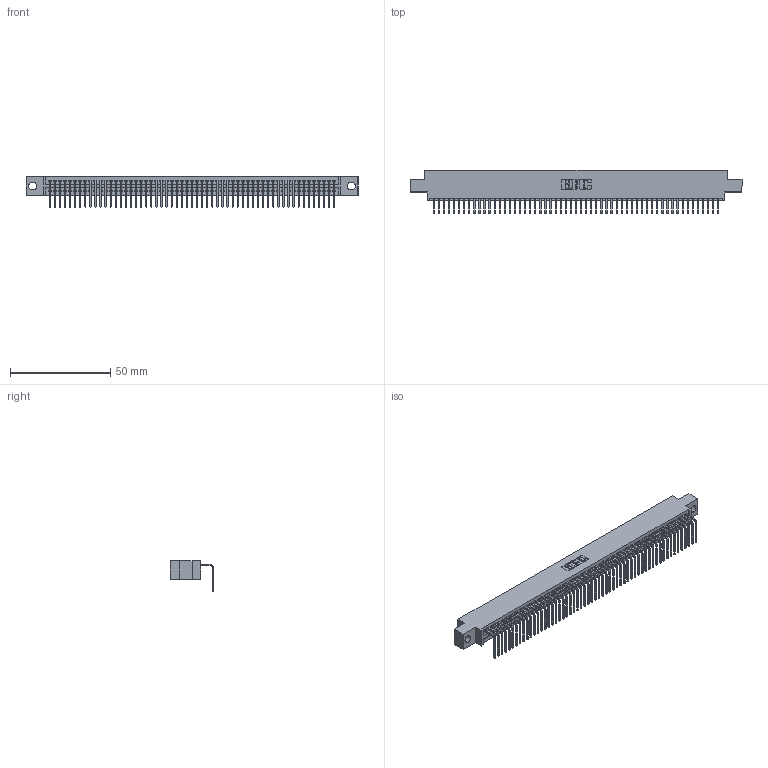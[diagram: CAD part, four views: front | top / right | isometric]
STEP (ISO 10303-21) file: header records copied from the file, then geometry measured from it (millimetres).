
FILE_DESCRIPTION (( 'STEP AP203' ), '1' );
FILE_NAME ('345-057-558-604.STEP', '2021-06-10T14:48:25', ( '' ), ( '' ), 'SwSTEP 2.0', 'SolidWorks 2020', '' );
FILE_SCHEMA (( 'CONFIG_CONTROL_DESIGN' ));
Length unit declared in the file: inch
Products named in the file (3): 345-057-558-604; 345 Part_0.170 Offset - 0.156 Dia-TI; 345-292-001_558 Tail - 2
Assembly tree (58 placements, depth 2):
  345-057-558-604
    345 Part_0.170 Offset - 0.156 Dia-TI
    345-292-001_558 Tail - 2  x57
Bounding box: 165.99 x 21.83 x 15.37 mm (x, y, z)
Volume: 15859.3 mm3; surface area: 22364.3 mm2
Topology: 58 solids, 58 shells, 3564 faces, 10763 edges, 7098 vertices
Faces by surface type: plane 2492, cylinder 1072
Entity records: 41515 total; most frequent: CARTESIAN_POINT 7201, ORIENTED_EDGE 7190, DIRECTION 6265, EDGE_CURVE 3595, VECTOR 3235, LINE 3235, VERTEX_POINT 2394, AXIS2_PLACEMENT_3D 1515
